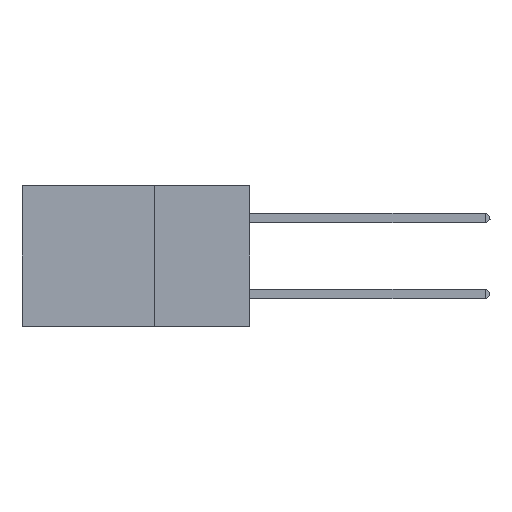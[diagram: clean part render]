
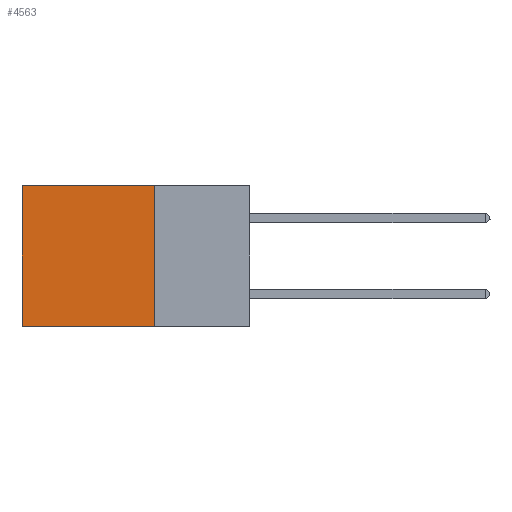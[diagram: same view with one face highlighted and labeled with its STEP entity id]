
A CAD part, left-side view. The second image highlights one B-rep face of the part: STEP entity #4563.
In plain terms, the highlighted planar face has unit normal (-1, 0, 0).
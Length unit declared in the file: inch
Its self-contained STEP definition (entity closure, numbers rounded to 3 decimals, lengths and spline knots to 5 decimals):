
#418 = LINE ( 'NONE', #11471, #2902 ) ;
#1078 = LINE ( 'NONE', #5574, #1407 ) ;
#1407 = VECTOR ( 'NONE', #2043, 39.37008 ) ;
#2043 = DIRECTION ( 'NONE',  ( 0., 1., 0. ) ) ;
#2760 = CARTESIAN_POINT ( 'NONE',  ( 0.2875, 0.25, 0. ) ) ;
#2902 = VECTOR ( 'NONE', #5856, 39.37008 ) ;
#3085 = ORIENTED_EDGE ( 'NONE', *, *, #5786, .F. ) ;
#3101 = VERTEX_POINT ( 'NONE', #4757 ) ;
#3370 = PLANE ( 'NONE',  #11857 ) ;
#3443 = FACE_OUTER_BOUND ( 'NONE', #3637, .T. ) ;
#3637 = EDGE_LOOP ( 'NONE', ( #11902, #3085, #4603, #12257 ) ) ;
#4121 = CARTESIAN_POINT ( 'NONE',  ( 0.2875, 0.6, 0. ) ) ;
#4310 = VECTOR ( 'NONE', #13956, 39.37008 ) ;
#4509 = CARTESIAN_POINT ( 'NONE',  ( 0.2875, 0.25, -0.37 ) ) ;
#4563 = ADVANCED_FACE ( 'NONE', ( #3443 ), #3370, .F. ) ;
#4603 = ORIENTED_EDGE ( 'NONE', *, *, #5345, .F. ) ;
#4654 = LINE ( 'NONE', #9134, #6544 ) ;
#4757 = CARTESIAN_POINT ( 'NONE',  ( 0.2875, 0.6, -0.37 ) ) ;
#5345 = EDGE_CURVE ( 'NONE', #9814, #8218, #4654, .T. ) ;
#5574 = CARTESIAN_POINT ( 'NONE',  ( 0.2875, 0.25, -0.37 ) ) ;
#5627 = VERTEX_POINT ( 'NONE', #4121 ) ;
#5786 = EDGE_CURVE ( 'NONE', #8218, #3101, #1078, .T. ) ;
#5856 = DIRECTION ( 'NONE',  ( 0., 0., -1. ) ) ;
#6544 = VECTOR ( 'NONE', #13558, 39.37008 ) ;
#7375 = CARTESIAN_POINT ( 'NONE',  ( 0.2875, 0.25, 0. ) ) ;
#8218 = VERTEX_POINT ( 'NONE', #4509 ) ;
#8742 = CARTESIAN_POINT ( 'NONE',  ( 0.2875, 0.25, 0. ) ) ;
#9134 = CARTESIAN_POINT ( 'NONE',  ( 0.2875, 0.25, 0. ) ) ;
#9467 = LINE ( 'NONE', #2760, #4310 ) ;
#9814 = VERTEX_POINT ( 'NONE', #7375 ) ;
#9860 = DIRECTION ( 'NONE',  ( 0., 0., -1. ) ) ;
#11471 = CARTESIAN_POINT ( 'NONE',  ( 0.2875, 0.6, 0. ) ) ;
#11473 = EDGE_CURVE ( 'NONE', #5627, #3101, #418, .T. ) ;
#11857 = AXIS2_PLACEMENT_3D ( 'NONE', #8742, #12370, #9860 ) ;
#11902 = ORIENTED_EDGE ( 'NONE', *, *, #11473, .T. ) ;
#12257 = ORIENTED_EDGE ( 'NONE', *, *, #13376, .T. ) ;
#12370 = DIRECTION ( 'NONE',  ( 1., 0., 0. ) ) ;
#13376 = EDGE_CURVE ( 'NONE', #9814, #5627, #9467, .T. ) ;
#13558 = DIRECTION ( 'NONE',  ( 0., 0., -1. ) ) ;
#13956 = DIRECTION ( 'NONE',  ( 0., 1., 0. ) ) ;
